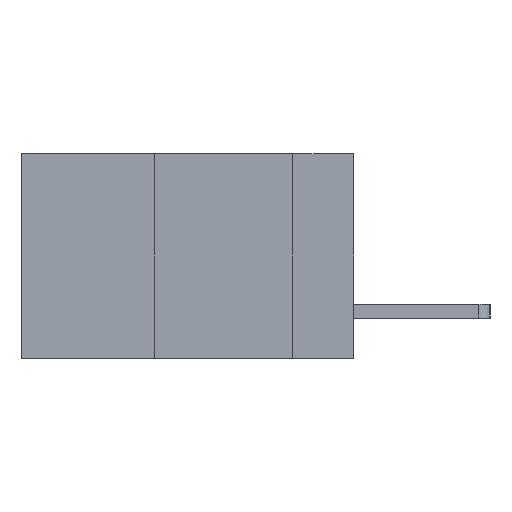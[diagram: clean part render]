
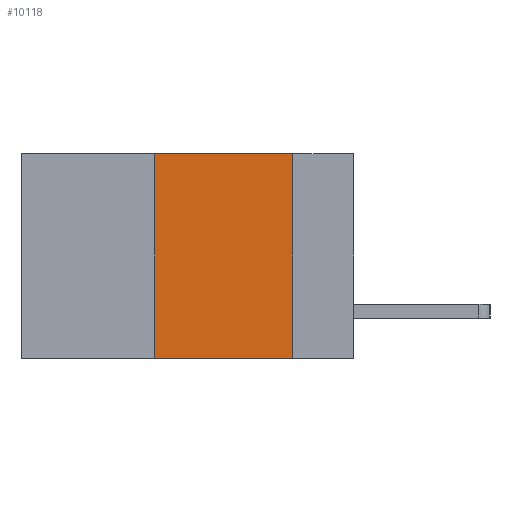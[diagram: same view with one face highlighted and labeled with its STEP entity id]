
A CAD part, left-side view. The second image highlights one B-rep face of the part: STEP entity #10118.
In plain terms, the highlighted planar face has unit normal (-1, 0, 0).
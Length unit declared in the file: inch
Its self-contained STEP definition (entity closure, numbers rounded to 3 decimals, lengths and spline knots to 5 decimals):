
#21 = DIRECTION ( 'NONE',  ( 0., 0., -1. ) ) ;
#296 = EDGE_CURVE ( 'NONE', #9022, #7447, #636, .T. ) ;
#406 = AXIS2_PLACEMENT_3D ( 'NONE', #12376, #6312, #10569 ) ;
#603 = VECTOR ( 'NONE', #10950, 39.37008 ) ;
#636 = LINE ( 'NONE', #5988, #3744 ) ;
#1119 = EDGE_LOOP ( 'NONE', ( #9454, #7346, #8999, #6961 ) ) ;
#2465 = LINE ( 'NONE', #4644, #10825 ) ;
#3744 = VECTOR ( 'NONE', #8082, 39.37008 ) ;
#4644 = CARTESIAN_POINT ( 'NONE',  ( 0., 0.6, 0. ) ) ;
#5319 = VERTEX_POINT ( 'NONE', #10027 ) ;
#5988 = CARTESIAN_POINT ( 'NONE',  ( 0., 0.6, -0.37 ) ) ;
#6312 = DIRECTION ( 'NONE',  ( 1., 0., 0. ) ) ;
#6803 = DIRECTION ( 'NONE',  ( 0., -1., 0. ) ) ;
#6961 = ORIENTED_EDGE ( 'NONE', *, *, #296, .T. ) ;
#7247 = FACE_OUTER_BOUND ( 'NONE', #1119, .T. ) ;
#7346 = ORIENTED_EDGE ( 'NONE', *, *, #9017, .F. ) ;
#7447 = VERTEX_POINT ( 'NONE', #7985 ) ;
#7985 = CARTESIAN_POINT ( 'NONE',  ( 0., 0.11, -0.37 ) ) ;
#8082 = DIRECTION ( 'NONE',  ( 0., -1., 0. ) ) ;
#8140 = PLANE ( 'NONE',  #406 ) ;
#8444 = LINE ( 'NONE', #11622, #12421 ) ;
#8613 = LINE ( 'NONE', #8678, #603 ) ;
#8678 = CARTESIAN_POINT ( 'NONE',  ( 0., 0.36, 0. ) ) ;
#8999 = ORIENTED_EDGE ( 'NONE', *, *, #9055, .F. ) ;
#9017 = EDGE_CURVE ( 'NONE', #5319, #11746, #2465, .T. ) ;
#9022 = VERTEX_POINT ( 'NONE', #9919 ) ;
#9055 = EDGE_CURVE ( 'NONE', #9022, #5319, #8613, .T. ) ;
#9454 = ORIENTED_EDGE ( 'NONE', *, *, #10934, .F. ) ;
#9919 = CARTESIAN_POINT ( 'NONE',  ( 0., 0.36, -0.37 ) ) ;
#10027 = CARTESIAN_POINT ( 'NONE',  ( 0., 0.36, 0. ) ) ;
#10118 = ADVANCED_FACE ( 'NONE', ( #7247 ), #8140, .F. ) ;
#10569 = DIRECTION ( 'NONE',  ( 0., 0., -1. ) ) ;
#10825 = VECTOR ( 'NONE', #6803, 39.37008 ) ;
#10934 = EDGE_CURVE ( 'NONE', #11746, #7447, #8444, .T. ) ;
#10950 = DIRECTION ( 'NONE',  ( 0., 0., 1. ) ) ;
#11622 = CARTESIAN_POINT ( 'NONE',  ( 0., 0.11, 0. ) ) ;
#11746 = VERTEX_POINT ( 'NONE', #13478 ) ;
#12376 = CARTESIAN_POINT ( 'NONE',  ( 0., 0.6, 0. ) ) ;
#12421 = VECTOR ( 'NONE', #21, 39.37008 ) ;
#13478 = CARTESIAN_POINT ( 'NONE',  ( 0., 0.11, 0. ) ) ;
